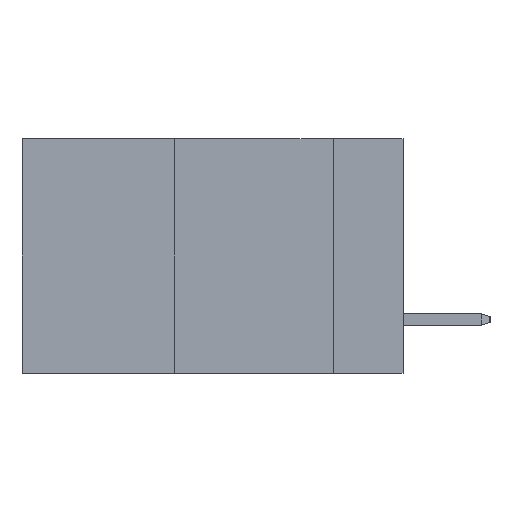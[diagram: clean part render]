
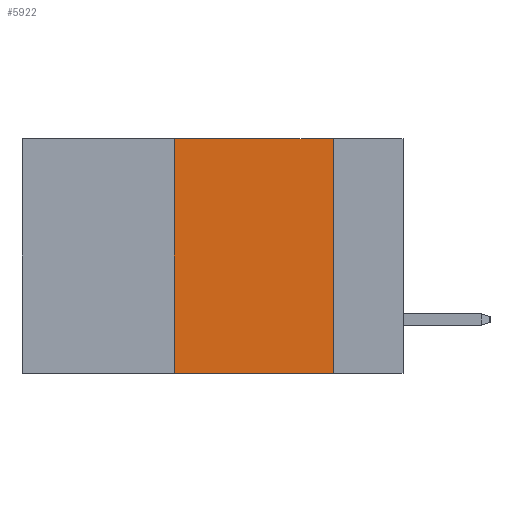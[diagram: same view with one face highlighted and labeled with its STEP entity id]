
A CAD part, left-side view. The second image highlights one B-rep face of the part: STEP entity #5922.
In plain terms, the highlighted planar face has unit normal (-1, 0, 0).
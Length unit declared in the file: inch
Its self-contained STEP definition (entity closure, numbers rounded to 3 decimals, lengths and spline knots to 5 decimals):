
#555 = CARTESIAN_POINT ( 'NONE',  ( 0., 0.11, 0. ) ) ;
#1091 = CARTESIAN_POINT ( 'NONE',  ( 0., 0.36, -0.37 ) ) ;
#1227 = CARTESIAN_POINT ( 'NONE',  ( 0., 0.6, 0. ) ) ;
#1562 = EDGE_CURVE ( 'NONE', #6825, #4492, #11900, .T. ) ;
#1848 = PLANE ( 'NONE',  #2132 ) ;
#1918 = CARTESIAN_POINT ( 'NONE',  ( 0., 0.6, 0. ) ) ;
#2042 = DIRECTION ( 'NONE',  ( 0., 0., -1. ) ) ;
#2132 = AXIS2_PLACEMENT_3D ( 'NONE', #1918, #2878, #2042 ) ;
#2189 = DIRECTION ( 'NONE',  ( 0., -1., 0. ) ) ;
#2265 = ORIENTED_EDGE ( 'NONE', *, *, #5617, .T. ) ;
#2878 = DIRECTION ( 'NONE',  ( 1., 0., 0. ) ) ;
#2958 = CARTESIAN_POINT ( 'NONE',  ( 0., 0.11, -0.37 ) ) ;
#3188 = LINE ( 'NONE', #7066, #5185 ) ;
#3525 = DIRECTION ( 'NONE',  ( 0., -1., 0. ) ) ;
#3907 = EDGE_LOOP ( 'NONE', ( #11363, #11554, #10352, #2265 ) ) ;
#4492 = VERTEX_POINT ( 'NONE', #555 ) ;
#4691 = VECTOR ( 'NONE', #9565, 39.37008 ) ;
#5177 = VECTOR ( 'NONE', #2189, 39.37008 ) ;
#5185 = VECTOR ( 'NONE', #10975, 39.37008 ) ;
#5617 = EDGE_CURVE ( 'NONE', #11604, #6654, #7022, .T. ) ;
#5922 = ADVANCED_FACE ( 'NONE', ( #10588 ), #1848, .F. ) ;
#6042 = EDGE_CURVE ( 'NONE', #4492, #6654, #3188, .T. ) ;
#6654 = VERTEX_POINT ( 'NONE', #2958 ) ;
#6825 = VERTEX_POINT ( 'NONE', #8486 ) ;
#7022 = LINE ( 'NONE', #10923, #5177 ) ;
#7066 = CARTESIAN_POINT ( 'NONE',  ( 0., 0.11, 0. ) ) ;
#8102 = VECTOR ( 'NONE', #3525, 39.37008 ) ;
#8486 = CARTESIAN_POINT ( 'NONE',  ( 0., 0.36, 0. ) ) ;
#8621 = CARTESIAN_POINT ( 'NONE',  ( 0., 0.36, 0. ) ) ;
#8684 = LINE ( 'NONE', #8621, #4691 ) ;
#9098 = EDGE_CURVE ( 'NONE', #11604, #6825, #8684, .T. ) ;
#9565 = DIRECTION ( 'NONE',  ( 0., 0., 1. ) ) ;
#10352 = ORIENTED_EDGE ( 'NONE', *, *, #9098, .F. ) ;
#10588 = FACE_OUTER_BOUND ( 'NONE', #3907, .T. ) ;
#10923 = CARTESIAN_POINT ( 'NONE',  ( 0., 0.6, -0.37 ) ) ;
#10975 = DIRECTION ( 'NONE',  ( 0., 0., -1. ) ) ;
#11363 = ORIENTED_EDGE ( 'NONE', *, *, #6042, .F. ) ;
#11554 = ORIENTED_EDGE ( 'NONE', *, *, #1562, .F. ) ;
#11604 = VERTEX_POINT ( 'NONE', #1091 ) ;
#11900 = LINE ( 'NONE', #1227, #8102 ) ;
